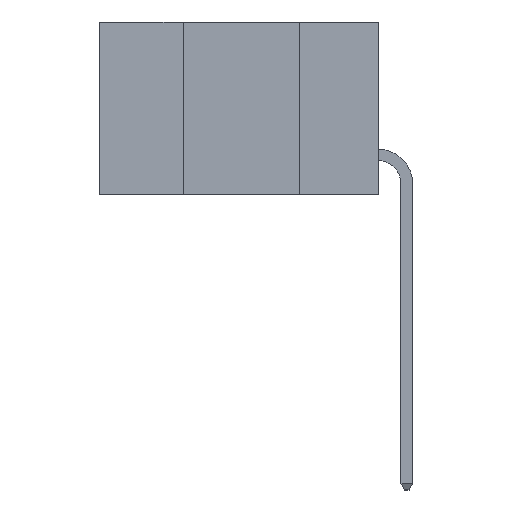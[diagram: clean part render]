
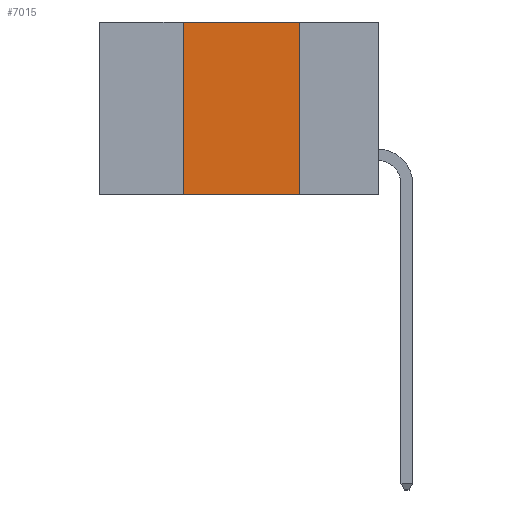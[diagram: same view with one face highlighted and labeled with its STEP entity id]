
A CAD part, left-side view. The second image highlights one B-rep face of the part: STEP entity #7015.
In plain terms, the highlighted planar face has unit normal (-1, 0, 0).
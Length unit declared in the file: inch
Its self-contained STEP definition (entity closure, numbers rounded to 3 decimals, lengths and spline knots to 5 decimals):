
#982 = LINE ( 'NONE', #5479, #4010 ) ;
#1975 = CARTESIAN_POINT ( 'NONE',  ( 0., 0.42, -0.37 ) ) ;
#4010 = VECTOR ( 'NONE', #4308, 39.37008 ) ;
#4308 = DIRECTION ( 'NONE',  ( 0., -1., 0. ) ) ;
#4439 = CARTESIAN_POINT ( 'NONE',  ( 0., 0.6, -0.37 ) ) ;
#4774 = VECTOR ( 'NONE', #14989, 39.37008 ) ;
#4791 = DIRECTION ( 'NONE',  ( 1., 0., 0. ) ) ;
#5389 = VERTEX_POINT ( 'NONE', #5953 ) ;
#5479 = CARTESIAN_POINT ( 'NONE',  ( 0., 0.6, 0. ) ) ;
#5648 = DIRECTION ( 'NONE',  ( 0., -1., 0. ) ) ;
#5953 = CARTESIAN_POINT ( 'NONE',  ( 0., 0.17, -0.37 ) ) ;
#5991 = VERTEX_POINT ( 'NONE', #10172 ) ;
#6165 = CARTESIAN_POINT ( 'NONE',  ( 0., 0.42, 0. ) ) ;
#6285 = LINE ( 'NONE', #4439, #15888 ) ;
#6506 = EDGE_CURVE ( 'NONE', #14526, #10100, #8874, .T. ) ;
#7015 = ADVANCED_FACE ( 'NONE', ( #14408 ), #12321, .F. ) ;
#8151 = EDGE_CURVE ( 'NONE', #14526, #5389, #6285, .T. ) ;
#8483 = VECTOR ( 'NONE', #9034, 39.37008 ) ;
#8874 = LINE ( 'NONE', #9806, #8483 ) ;
#9034 = DIRECTION ( 'NONE',  ( 0., 0., 1. ) ) ;
#9788 = EDGE_LOOP ( 'NONE', ( #9862, #13646, #11097, #11507 ) ) ;
#9806 = CARTESIAN_POINT ( 'NONE',  ( 0., 0.42, -0.37 ) ) ;
#9862 = ORIENTED_EDGE ( 'NONE', *, *, #10751, .F. ) ;
#10100 = VERTEX_POINT ( 'NONE', #6165 ) ;
#10172 = CARTESIAN_POINT ( 'NONE',  ( 0., 0.17, 0. ) ) ;
#10751 = EDGE_CURVE ( 'NONE', #5991, #5389, #14744, .T. ) ;
#11097 = ORIENTED_EDGE ( 'NONE', *, *, #6506, .F. ) ;
#11507 = ORIENTED_EDGE ( 'NONE', *, *, #8151, .T. ) ;
#12321 = PLANE ( 'NONE',  #14658 ) ;
#12525 = CARTESIAN_POINT ( 'NONE',  ( 0., 0.17, -0.37 ) ) ;
#13557 = DIRECTION ( 'NONE',  ( 0., 0., -1. ) ) ;
#13646 = ORIENTED_EDGE ( 'NONE', *, *, #16041, .F. ) ;
#14408 = FACE_OUTER_BOUND ( 'NONE', #9788, .T. ) ;
#14526 = VERTEX_POINT ( 'NONE', #1975 ) ;
#14658 = AXIS2_PLACEMENT_3D ( 'NONE', #15951, #4791, #13557 ) ;
#14744 = LINE ( 'NONE', #12525, #4774 ) ;
#14989 = DIRECTION ( 'NONE',  ( 0., 0., -1. ) ) ;
#15888 = VECTOR ( 'NONE', #5648, 39.37008 ) ;
#15951 = CARTESIAN_POINT ( 'NONE',  ( 0., 0.6, 0. ) ) ;
#16041 = EDGE_CURVE ( 'NONE', #10100, #5991, #982, .T. ) ;
